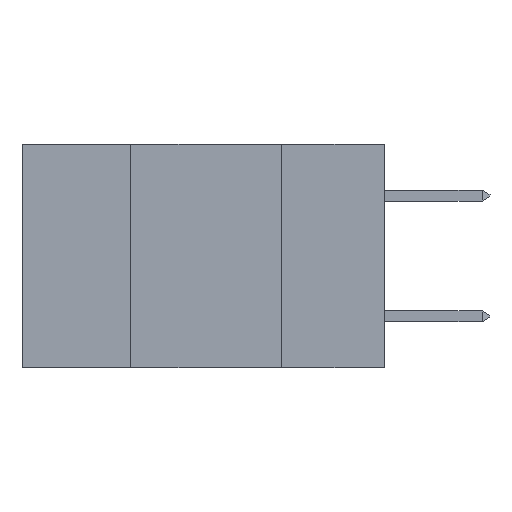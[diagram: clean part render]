
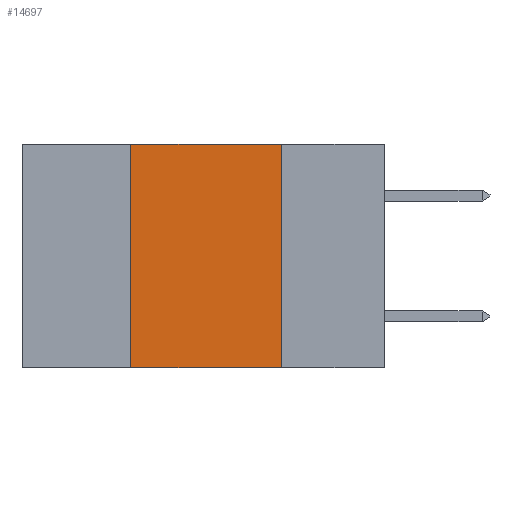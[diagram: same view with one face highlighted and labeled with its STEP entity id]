
A CAD part, left-side view. The second image highlights one B-rep face of the part: STEP entity #14697.
In plain terms, the highlighted planar face has unit normal (-1, 0, 0).
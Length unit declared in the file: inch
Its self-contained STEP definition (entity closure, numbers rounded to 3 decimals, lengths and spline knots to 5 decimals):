
#470 = VERTEX_POINT ( 'NONE', #9074 ) ;
#560 = VECTOR ( 'NONE', #2968, 39.37008 ) ;
#1152 = DIRECTION ( 'NONE',  ( 0., 0., -1. ) ) ;
#1215 = LINE ( 'NONE', #10200, #9135 ) ;
#1286 = AXIS2_PLACEMENT_3D ( 'NONE', #8179, #15244, #13594 ) ;
#1944 = CARTESIAN_POINT ( 'NONE',  ( 0., 0.17, -0.37 ) ) ;
#2968 = DIRECTION ( 'NONE',  ( 0., -1., 0. ) ) ;
#4231 = CARTESIAN_POINT ( 'NONE',  ( 0., 0.42, 0. ) ) ;
#5239 = FACE_OUTER_BOUND ( 'NONE', #7313, .T. ) ;
#5613 = ORIENTED_EDGE ( 'NONE', *, *, #9509, .F. ) ;
#6603 = ORIENTED_EDGE ( 'NONE', *, *, #12973, .F. ) ;
#6786 = LINE ( 'NONE', #8166, #17381 ) ;
#7313 = EDGE_LOOP ( 'NONE', ( #6603, #5613, #12267, #13766 ) ) ;
#8065 = LINE ( 'NONE', #12877, #560 ) ;
#8166 = CARTESIAN_POINT ( 'NONE',  ( 0., 0.17, 0. ) ) ;
#8179 = CARTESIAN_POINT ( 'NONE',  ( 0., 0.6, 0. ) ) ;
#9074 = CARTESIAN_POINT ( 'NONE',  ( 0., 0.42, -0.37 ) ) ;
#9135 = VECTOR ( 'NONE', #10320, 39.37008 ) ;
#9509 = EDGE_CURVE ( 'NONE', #13637, #14611, #1215, .T. ) ;
#9833 = EDGE_CURVE ( 'NONE', #470, #13637, #16842, .T. ) ;
#10200 = CARTESIAN_POINT ( 'NONE',  ( 0., 0.6, 0. ) ) ;
#10320 = DIRECTION ( 'NONE',  ( 0., -1., 0. ) ) ;
#10344 = CARTESIAN_POINT ( 'NONE',  ( 0., 0.42, 0. ) ) ;
#11954 = VECTOR ( 'NONE', #17505, 39.37008 ) ;
#12267 = ORIENTED_EDGE ( 'NONE', *, *, #9833, .F. ) ;
#12392 = PLANE ( 'NONE',  #1286 ) ;
#12877 = CARTESIAN_POINT ( 'NONE',  ( 0., 0.6, -0.37 ) ) ;
#12973 = EDGE_CURVE ( 'NONE', #14611, #15079, #6786, .T. ) ;
#13404 = CARTESIAN_POINT ( 'NONE',  ( 0., 0.17, 0. ) ) ;
#13594 = DIRECTION ( 'NONE',  ( 0., 0., -1. ) ) ;
#13637 = VERTEX_POINT ( 'NONE', #4231 ) ;
#13766 = ORIENTED_EDGE ( 'NONE', *, *, #16625, .T. ) ;
#14611 = VERTEX_POINT ( 'NONE', #13404 ) ;
#14697 = ADVANCED_FACE ( 'NONE', ( #5239 ), #12392, .F. ) ;
#15079 = VERTEX_POINT ( 'NONE', #1944 ) ;
#15244 = DIRECTION ( 'NONE',  ( 1., 0., 0. ) ) ;
#16625 = EDGE_CURVE ( 'NONE', #470, #15079, #8065, .T. ) ;
#16842 = LINE ( 'NONE', #10344, #11954 ) ;
#17381 = VECTOR ( 'NONE', #1152, 39.37008 ) ;
#17505 = DIRECTION ( 'NONE',  ( 0., 0., 1. ) ) ;
